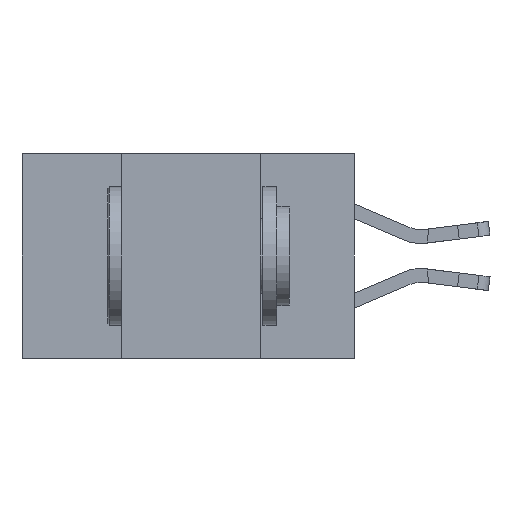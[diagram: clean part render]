
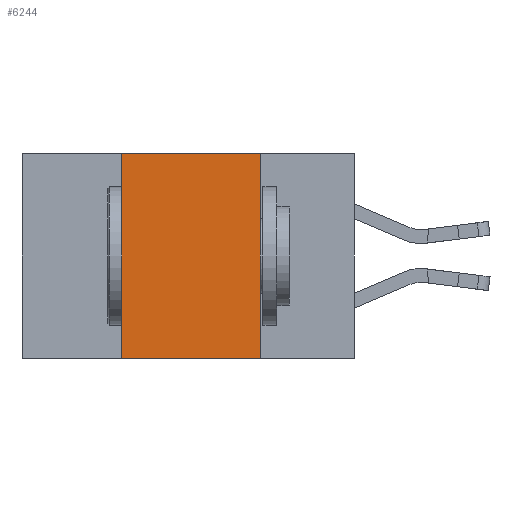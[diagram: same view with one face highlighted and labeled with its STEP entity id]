
A CAD part, left-side view. The second image highlights one B-rep face of the part: STEP entity #6244.
In plain terms, the highlighted planar face has unit normal (-1, 0, 0).
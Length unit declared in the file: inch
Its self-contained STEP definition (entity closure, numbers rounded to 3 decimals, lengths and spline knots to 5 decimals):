
#377 = DIRECTION ( 'NONE',  ( 1., 0., 0. ) ) ;
#765 = CARTESIAN_POINT ( 'NONE',  ( 0., 0.42, 0. ) ) ;
#915 = CARTESIAN_POINT ( 'NONE',  ( 0., 0.17, -0.37 ) ) ;
#1093 = DIRECTION ( 'NONE',  ( 0., -1., 0. ) ) ;
#1642 = CARTESIAN_POINT ( 'NONE',  ( 0., 0.17, 0. ) ) ;
#2192 = VECTOR ( 'NONE', #3771, 39.37008 ) ;
#2391 = EDGE_LOOP ( 'NONE', ( #16523, #10645, #17448, #15670 ) ) ;
#3319 = EDGE_CURVE ( 'NONE', #16270, #14082, #12091, .T. ) ;
#3595 = VERTEX_POINT ( 'NONE', #1642 ) ;
#3677 = CARTESIAN_POINT ( 'NONE',  ( 0., 0.6, 0. ) ) ;
#3763 = VECTOR ( 'NONE', #1093, 39.37008 ) ;
#3771 = DIRECTION ( 'NONE',  ( 0., 0., -1. ) ) ;
#3866 = CARTESIAN_POINT ( 'NONE',  ( 0., 0.42, -0.37 ) ) ;
#4306 = VECTOR ( 'NONE', #7090, 39.37008 ) ;
#5096 = CARTESIAN_POINT ( 'NONE',  ( 0., 0.17, 0. ) ) ;
#5207 = VERTEX_POINT ( 'NONE', #5460 ) ;
#5460 = CARTESIAN_POINT ( 'NONE',  ( 0., 0.42, 0. ) ) ;
#6187 = CARTESIAN_POINT ( 'NONE',  ( 0., 0.6, -0.37 ) ) ;
#6244 = ADVANCED_FACE ( 'NONE', ( #20219 ), #8845, .F. ) ;
#7090 = DIRECTION ( 'NONE',  ( 0., 0., 1. ) ) ;
#8389 = AXIS2_PLACEMENT_3D ( 'NONE', #3677, #377, #15363 ) ;
#8675 = EDGE_CURVE ( 'NONE', #16270, #5207, #8715, .T. ) ;
#8715 = LINE ( 'NONE', #765, #4306 ) ;
#8845 = PLANE ( 'NONE',  #8389 ) ;
#9356 = LINE ( 'NONE', #16391, #11156 ) ;
#10645 = ORIENTED_EDGE ( 'NONE', *, *, #13096, .F. ) ;
#11156 = VECTOR ( 'NONE', #18052, 39.37008 ) ;
#12091 = LINE ( 'NONE', #6187, #3763 ) ;
#13096 = EDGE_CURVE ( 'NONE', #5207, #3595, #9356, .T. ) ;
#14082 = VERTEX_POINT ( 'NONE', #915 ) ;
#15363 = DIRECTION ( 'NONE',  ( 0., 0., -1. ) ) ;
#15670 = ORIENTED_EDGE ( 'NONE', *, *, #3319, .T. ) ;
#16270 = VERTEX_POINT ( 'NONE', #3866 ) ;
#16391 = CARTESIAN_POINT ( 'NONE',  ( 0., 0.6, 0. ) ) ;
#16523 = ORIENTED_EDGE ( 'NONE', *, *, #16550, .F. ) ;
#16550 = EDGE_CURVE ( 'NONE', #3595, #14082, #17757, .T. ) ;
#17448 = ORIENTED_EDGE ( 'NONE', *, *, #8675, .F. ) ;
#17757 = LINE ( 'NONE', #5096, #2192 ) ;
#18052 = DIRECTION ( 'NONE',  ( 0., -1., 0. ) ) ;
#20219 = FACE_OUTER_BOUND ( 'NONE', #2391, .T. ) ;
